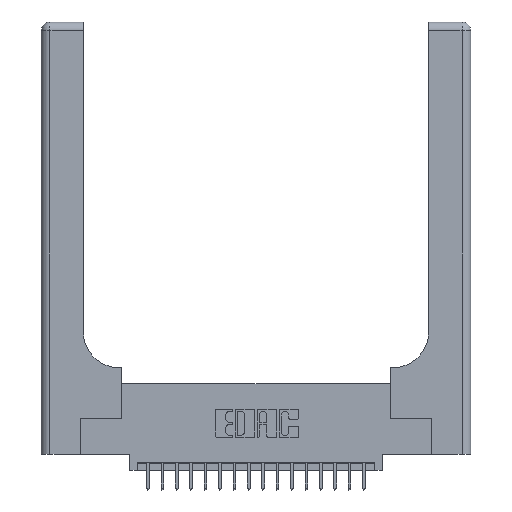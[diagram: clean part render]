
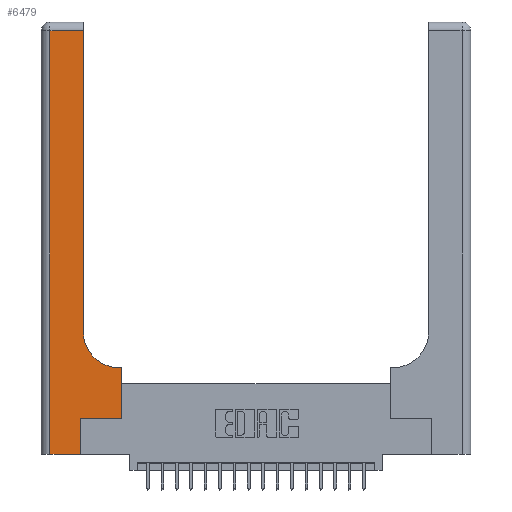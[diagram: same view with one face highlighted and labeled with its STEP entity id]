
A CAD part, top view. The second image highlights one B-rep face of the part: STEP entity #6479.
In plain terms, the highlighted planar face has unit normal (0, 0, 1).
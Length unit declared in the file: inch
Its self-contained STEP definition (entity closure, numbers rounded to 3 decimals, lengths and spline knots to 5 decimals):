
#36 = CARTESIAN_POINT ( 'NONE',  ( 0.2915, 3., 0.37 ) ) ;
#203 = CARTESIAN_POINT ( 'NONE',  ( 0.06, 2.94, 0.37 ) ) ;
#254 = CARTESIAN_POINT ( 'NONE',  ( 0.2915, 0.6, 0.37 ) ) ;
#765 = VERTEX_POINT ( 'NONE', #7091 ) ;
#844 = VECTOR ( 'NONE', #13494, 39.37008 ) ;
#941 = CARTESIAN_POINT ( 'NONE',  ( 0.269, 0., 0.37 ) ) ;
#1215 = LINE ( 'NONE', #19770, #14892 ) ;
#1701 = ORIENTED_EDGE ( 'NONE', *, *, #20553, .T. ) ;
#1716 = ORIENTED_EDGE ( 'NONE', *, *, #19837, .T. ) ;
#2225 = CARTESIAN_POINT ( 'NONE',  ( 0., 3., 0.37 ) ) ;
#2260 = LINE ( 'NONE', #5419, #13891 ) ;
#2379 = EDGE_CURVE ( 'NONE', #765, #9111, #14894, .T. ) ;
#2487 = CARTESIAN_POINT ( 'NONE',  ( 0.269, 0.25, 0.37 ) ) ;
#3970 = PLANE ( 'NONE',  #20443 ) ;
#4179 = VECTOR ( 'NONE', #8538, 39.37008 ) ;
#4259 = EDGE_CURVE ( 'NONE', #18539, #765, #7951, .T. ) ;
#4279 = VERTEX_POINT ( 'NONE', #2487 ) ;
#4853 = VECTOR ( 'NONE', #6683, 39.37008 ) ;
#5003 = ORIENTED_EDGE ( 'NONE', *, *, #14904, .T. ) ;
#5419 = CARTESIAN_POINT ( 'NONE',  ( 0., 2.94, 0.37 ) ) ;
#5747 = DIRECTION ( 'NONE',  ( 1., 0., 0. ) ) ;
#6479 = ADVANCED_FACE ( 'NONE', ( #17070 ), #3970, .F. ) ;
#6683 = DIRECTION ( 'NONE',  ( 0., 1., 0. ) ) ;
#6788 = CARTESIAN_POINT ( 'NONE',  ( 0.5415, 0.6, 0.37 ) ) ;
#7091 = CARTESIAN_POINT ( 'NONE',  ( 0.2915, 0.85, 0.37 ) ) ;
#7229 = DIRECTION ( 'NONE',  ( -1., 0., 0. ) ) ;
#7442 = DIRECTION ( 'NONE',  ( 0., -1., 0. ) ) ;
#7575 = DIRECTION ( 'NONE',  ( 0., 1., 0. ) ) ;
#7619 = VECTOR ( 'NONE', #13831, 39.37008 ) ;
#7797 = CARTESIAN_POINT ( 'NONE',  ( 0.06, 0., 0.37 ) ) ;
#7951 = CIRCLE ( 'NONE', #15884, 0.25 ) ;
#8538 = DIRECTION ( 'NONE',  ( 1., 0., 0. ) ) ;
#9111 = VERTEX_POINT ( 'NONE', #12363 ) ;
#9137 = VERTEX_POINT ( 'NONE', #7797 ) ;
#9158 = EDGE_CURVE ( 'NONE', #20270, #4279, #14295, .T. ) ;
#9485 = CARTESIAN_POINT ( 'NONE',  ( 0.5585, 0.25, 0.37 ) ) ;
#9495 = VERTEX_POINT ( 'NONE', #10620 ) ;
#9861 = CARTESIAN_POINT ( 'NONE',  ( 0., 0., 0.37 ) ) ;
#10507 = CARTESIAN_POINT ( 'NONE',  ( 0.5585, 0.25, 0.37 ) ) ;
#10620 = CARTESIAN_POINT ( 'NONE',  ( 0.5585, 0.6, 0.37 ) ) ;
#10980 = ORIENTED_EDGE ( 'NONE', *, *, #11345, .T. ) ;
#11345 = EDGE_CURVE ( 'NONE', #15642, #9495, #15462, .T. ) ;
#11548 = DIRECTION ( 'NONE',  ( 1., 0., 0. ) ) ;
#11572 = LINE ( 'NONE', #9861, #4179 ) ;
#11631 = ORIENTED_EDGE ( 'NONE', *, *, #4259, .T. ) ;
#12132 = VECTOR ( 'NONE', #7442, 39.37008 ) ;
#12254 = DIRECTION ( 'NONE',  ( -1., 0., 0. ) ) ;
#12363 = CARTESIAN_POINT ( 'NONE',  ( 0.2915, 2.94, 0.37 ) ) ;
#13494 = DIRECTION ( 'NONE',  ( -1., 0., 0. ) ) ;
#13831 = DIRECTION ( 'NONE',  ( 0., 1., 0. ) ) ;
#13891 = VECTOR ( 'NONE', #12254, 39.37008 ) ;
#13952 = DIRECTION ( 'NONE',  ( 0., 0., -1. ) ) ;
#13991 = DIRECTION ( 'NONE',  ( 0., 0., -1. ) ) ;
#14295 = LINE ( 'NONE', #941, #19368 ) ;
#14443 = ORIENTED_EDGE ( 'NONE', *, *, #9158, .T. ) ;
#14858 = ORIENTED_EDGE ( 'NONE', *, *, #2379, .T. ) ;
#14892 = VECTOR ( 'NONE', #11548, 39.37008 ) ;
#14894 = LINE ( 'NONE', #36, #4853 ) ;
#14904 = EDGE_CURVE ( 'NONE', #9495, #18539, #15127, .T. ) ;
#15127 = LINE ( 'NONE', #254, #844 ) ;
#15462 = LINE ( 'NONE', #10507, #7619 ) ;
#15466 = LINE ( 'NONE', #20572, #12132 ) ;
#15611 = CARTESIAN_POINT ( 'NONE',  ( 0.5415, 0.85, 0.37 ) ) ;
#15642 = VERTEX_POINT ( 'NONE', #9485 ) ;
#15884 = AXIS2_PLACEMENT_3D ( 'NONE', #15611, #13991, #5747 ) ;
#16249 = CARTESIAN_POINT ( 'NONE',  ( 0.269, 0., 0.37 ) ) ;
#16440 = EDGE_CURVE ( 'NONE', #4279, #15642, #1215, .T. ) ;
#17070 = FACE_OUTER_BOUND ( 'NONE', #18451, .T. ) ;
#17669 = EDGE_CURVE ( 'NONE', #9137, #20270, #11572, .T. ) ;
#18451 = EDGE_LOOP ( 'NONE', ( #14858, #1701, #1716, #18786, #14443, #21271, #10980, #5003, #11631 ) ) ;
#18539 = VERTEX_POINT ( 'NONE', #6788 ) ;
#18786 = ORIENTED_EDGE ( 'NONE', *, *, #17669, .T. ) ;
#19368 = VECTOR ( 'NONE', #7575, 39.37008 ) ;
#19770 = CARTESIAN_POINT ( 'NONE',  ( 0.269, 0.25, 0.37 ) ) ;
#19837 = EDGE_CURVE ( 'NONE', #20398, #9137, #15466, .T. ) ;
#20270 = VERTEX_POINT ( 'NONE', #16249 ) ;
#20398 = VERTEX_POINT ( 'NONE', #203 ) ;
#20443 = AXIS2_PLACEMENT_3D ( 'NONE', #2225, #13952, #7229 ) ;
#20553 = EDGE_CURVE ( 'NONE', #9111, #20398, #2260, .T. ) ;
#20572 = CARTESIAN_POINT ( 'NONE',  ( 0.06, 3., 0.37 ) ) ;
#21271 = ORIENTED_EDGE ( 'NONE', *, *, #16440, .T. ) ;
